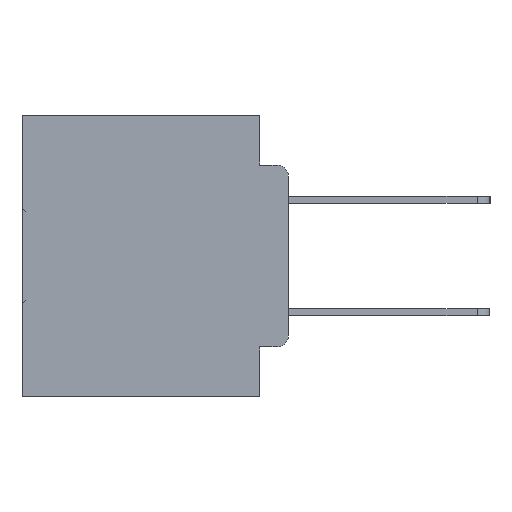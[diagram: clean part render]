
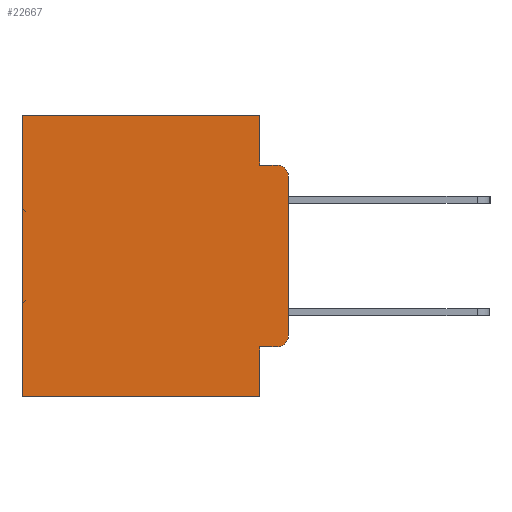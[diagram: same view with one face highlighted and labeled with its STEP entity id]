
A CAD part, left-side view. The second image highlights one B-rep face of the part: STEP entity #22667.
In plain terms, the highlighted planar face has unit normal (-1, 0, 0).
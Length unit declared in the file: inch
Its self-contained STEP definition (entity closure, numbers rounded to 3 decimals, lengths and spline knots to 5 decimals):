
#1205 = DIRECTION ( 'NONE',  ( 0., 1., 0. ) ) ;
#1636 = CARTESIAN_POINT ( 'NONE',  ( 0.298, 0., -0.3915 ) ) ;
#2065 = ORIENTED_EDGE ( 'NONE', *, *, #21849, .T. ) ;
#2132 = DIRECTION ( 'NONE',  ( -1., 0., 0. ) ) ;
#2214 = DIRECTION ( 'NONE',  ( 0., 0., -1. ) ) ;
#2322 = CARTESIAN_POINT ( 'NONE',  ( 0.298, 0.051, -0.4115 ) ) ;
#2573 = VECTOR ( 'NONE', #17569, 39.37008 ) ;
#3125 = VERTEX_POINT ( 'NONE', #18921 ) ;
#3538 = CARTESIAN_POINT ( 'NONE',  ( 0.298, 0.051, -0.4115 ) ) ;
#3883 = DIRECTION ( 'NONE',  ( 0., -1., 0. ) ) ;
#4302 = LINE ( 'NONE', #6926, #2573 ) ;
#4417 = EDGE_LOOP ( 'NONE', ( #10089, #25850, #21378, #27117, #31227, #2065, #5100, #17058, #24443, #31883 ) ) ;
#4810 = VERTEX_POINT ( 'NONE', #9483 ) ;
#5100 = ORIENTED_EDGE ( 'NONE', *, *, #28476, .F. ) ;
#5622 = CARTESIAN_POINT ( 'NONE',  ( 0.298, 0., 0. ) ) ;
#6278 = DIRECTION ( 'NONE',  ( 0., -1., 0. ) ) ;
#6926 = CARTESIAN_POINT ( 'NONE',  ( 0.298, 0.051, 0. ) ) ;
#7096 = CARTESIAN_POINT ( 'NONE',  ( 0.298, 0.051, 0. ) ) ;
#7492 = VERTEX_POINT ( 'NONE', #2322 ) ;
#7645 = EDGE_CURVE ( 'NONE', #12893, #9911, #19235, .T. ) ;
#7878 = LINE ( 'NONE', #31898, #8728 ) ;
#7910 = CARTESIAN_POINT ( 'NONE',  ( 0.298, 0., 0. ) ) ;
#8728 = VECTOR ( 'NONE', #18852, 39.37008 ) ;
#9483 = CARTESIAN_POINT ( 'NONE',  ( 0.298, 0.02, -0.4115 ) ) ;
#9911 = VERTEX_POINT ( 'NONE', #10769 ) ;
#10089 = ORIENTED_EDGE ( 'NONE', *, *, #15985, .F. ) ;
#10769 = CARTESIAN_POINT ( 'NONE',  ( 0.298, 0.473, 0. ) ) ;
#10979 = PLANE ( 'NONE',  #30957 ) ;
#12152 = CARTESIAN_POINT ( 'NONE',  ( 0.298, 0.02, -0.3915 ) ) ;
#12893 = VERTEX_POINT ( 'NONE', #18667 ) ;
#12930 = AXIS2_PLACEMENT_3D ( 'NONE', #12152, #30622, #14835 ) ;
#13022 = CARTESIAN_POINT ( 'NONE',  ( 0.298, 0.473, 0. ) ) ;
#13682 = DIRECTION ( 'NONE',  ( 0., 0., -1. ) ) ;
#14769 = LINE ( 'NONE', #22596, #15586 ) ;
#14835 = DIRECTION ( 'NONE',  ( 0., 0., -1. ) ) ;
#15060 = VERTEX_POINT ( 'NONE', #1636 ) ;
#15395 = CARTESIAN_POINT ( 'NONE',  ( 0.298, 0.051, -0.0885 ) ) ;
#15586 = VECTOR ( 'NONE', #3883, 39.37008 ) ;
#15985 = EDGE_CURVE ( 'NONE', #20615, #15060, #7878, .T. ) ;
#16775 = VERTEX_POINT ( 'NONE', #22154 ) ;
#17058 = ORIENTED_EDGE ( 'NONE', *, *, #23198, .F. ) ;
#17157 = DIRECTION ( 'NONE',  ( 0., 1., 0. ) ) ;
#17569 = DIRECTION ( 'NONE',  ( 0., 0., -1. ) ) ;
#18248 = CARTESIAN_POINT ( 'NONE',  ( 0.298, 0.02, -0.1085 ) ) ;
#18325 = VERTEX_POINT ( 'NONE', #22021 ) ;
#18399 = VECTOR ( 'NONE', #1205, 39.37008 ) ;
#18667 = CARTESIAN_POINT ( 'NONE',  ( 0.298, 0.051, 0. ) ) ;
#18852 = DIRECTION ( 'NONE',  ( 0., 0., -1. ) ) ;
#18921 = CARTESIAN_POINT ( 'NONE',  ( 0.298, 0.051, -0.5 ) ) ;
#19170 = EDGE_CURVE ( 'NONE', #4810, #15060, #31369, .T. ) ;
#19178 = VECTOR ( 'NONE', #6278, 39.37008 ) ;
#19235 = LINE ( 'NONE', #7910, #18399 ) ;
#19324 = EDGE_CURVE ( 'NONE', #20615, #16775, #27258, .T. ) ;
#20615 = VERTEX_POINT ( 'NONE', #34265 ) ;
#20911 = DIRECTION ( 'NONE',  ( 0., 0., -1. ) ) ;
#21378 = ORIENTED_EDGE ( 'NONE', *, *, #28482, .F. ) ;
#21849 = EDGE_CURVE ( 'NONE', #9911, #18325, #24219, .T. ) ;
#22021 = CARTESIAN_POINT ( 'NONE',  ( 0.298, 0.473, -0.5 ) ) ;
#22154 = CARTESIAN_POINT ( 'NONE',  ( 0.298, 0.02, -0.0885 ) ) ;
#22505 = LINE ( 'NONE', #7096, #29401 ) ;
#22596 = CARTESIAN_POINT ( 'NONE',  ( 0.298, 0.051, -0.0885 ) ) ;
#22667 = ADVANCED_FACE ( 'NONE', ( #31929 ), #10979, .F. ) ;
#22690 = LINE ( 'NONE', #30352, #28755 ) ;
#23044 = DIRECTION ( 'NONE',  ( 0., 0., -1. ) ) ;
#23198 = EDGE_CURVE ( 'NONE', #7492, #3125, #22505, .T. ) ;
#24219 = LINE ( 'NONE', #13022, #31992 ) ;
#24443 = ORIENTED_EDGE ( 'NONE', *, *, #24955, .T. ) ;
#24955 = EDGE_CURVE ( 'NONE', #7492, #4810, #33096, .T. ) ;
#25850 = ORIENTED_EDGE ( 'NONE', *, *, #19324, .T. ) ;
#27117 = ORIENTED_EDGE ( 'NONE', *, *, #33903, .F. ) ;
#27258 = CIRCLE ( 'NONE', #32402, 0.02 ) ;
#28048 = VERTEX_POINT ( 'NONE', #15395 ) ;
#28476 = EDGE_CURVE ( 'NONE', #3125, #18325, #22690, .T. ) ;
#28482 = EDGE_CURVE ( 'NONE', #28048, #16775, #14769, .T. ) ;
#28755 = VECTOR ( 'NONE', #17157, 39.37008 ) ;
#29401 = VECTOR ( 'NONE', #23044, 39.37008 ) ;
#29471 = DIRECTION ( 'NONE',  ( 1., 0., 0. ) ) ;
#30352 = CARTESIAN_POINT ( 'NONE',  ( 0.298, 0., -0.5 ) ) ;
#30622 = DIRECTION ( 'NONE',  ( -1., 0., 0. ) ) ;
#30957 = AXIS2_PLACEMENT_3D ( 'NONE', #5622, #29471, #13682 ) ;
#31227 = ORIENTED_EDGE ( 'NONE', *, *, #7645, .T. ) ;
#31369 = CIRCLE ( 'NONE', #12930, 0.02 ) ;
#31883 = ORIENTED_EDGE ( 'NONE', *, *, #19170, .T. ) ;
#31898 = CARTESIAN_POINT ( 'NONE',  ( 0.298, 0., 0. ) ) ;
#31929 = FACE_OUTER_BOUND ( 'NONE', #4417, .T. ) ;
#31992 = VECTOR ( 'NONE', #2214, 39.37008 ) ;
#32402 = AXIS2_PLACEMENT_3D ( 'NONE', #18248, #2132, #20911 ) ;
#33096 = LINE ( 'NONE', #3538, #19178 ) ;
#33903 = EDGE_CURVE ( 'NONE', #12893, #28048, #4302, .T. ) ;
#34265 = CARTESIAN_POINT ( 'NONE',  ( 0.298, 0., -0.1085 ) ) ;
